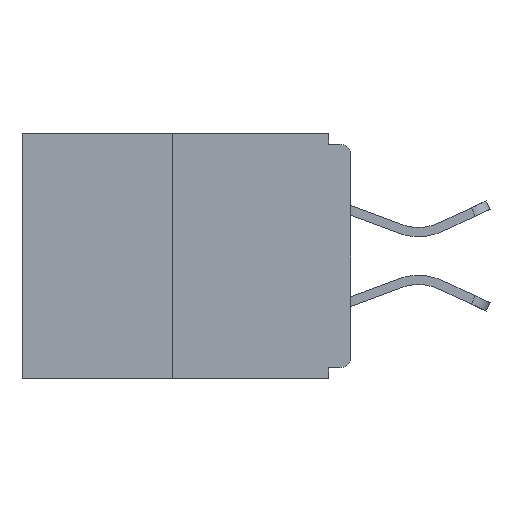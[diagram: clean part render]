
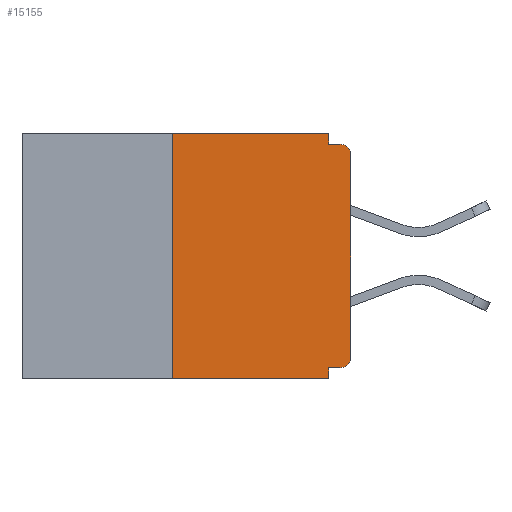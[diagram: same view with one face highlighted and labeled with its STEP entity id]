
A CAD part, left-side view. The second image highlights one B-rep face of the part: STEP entity #15155.
In plain terms, the highlighted planar face has unit normal (-1, 0, 0).
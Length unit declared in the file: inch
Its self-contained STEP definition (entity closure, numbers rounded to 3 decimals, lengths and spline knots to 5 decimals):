
#83 = CARTESIAN_POINT ( 'NONE',  ( 0., 0.015, -0.03 ) ) ;
#895 = CARTESIAN_POINT ( 'NONE',  ( 0., 0.46, 0. ) ) ;
#1027 = VECTOR ( 'NONE', #2472, 39.37008 ) ;
#1041 = VERTEX_POINT ( 'NONE', #11743 ) ;
#1158 = CARTESIAN_POINT ( 'NONE',  ( 0., 0.015, -0.328 ) ) ;
#1202 = FACE_OUTER_BOUND ( 'NONE', #19385, .T. ) ;
#1250 = LINE ( 'NONE', #4895, #5093 ) ;
#1972 = EDGE_CURVE ( 'NONE', #18766, #8095, #3754, .T. ) ;
#2022 = DIRECTION ( 'NONE',  ( -1., 0., 0. ) ) ;
#2089 = VECTOR ( 'NONE', #27656, 39.37008 ) ;
#2280 = ORIENTED_EDGE ( 'NONE', *, *, #21672, .F. ) ;
#2422 = DIRECTION ( 'NONE',  ( 0., 0., -1. ) ) ;
#2425 = LINE ( 'NONE', #4807, #1027 ) ;
#2444 = AXIS2_PLACEMENT_3D ( 'NONE', #895, #22980, #5081 ) ;
#2463 = VECTOR ( 'NONE', #12891, 39.37008 ) ;
#2472 = DIRECTION ( 'NONE',  ( 0., 0., 1. ) ) ;
#2702 = CARTESIAN_POINT ( 'NONE',  ( 0., 0., 0. ) ) ;
#3128 = PLANE ( 'NONE',  #2444 ) ;
#3177 = VECTOR ( 'NONE', #22020, 39.37008 ) ;
#3754 = LINE ( 'NONE', #13564, #22921 ) ;
#3843 = VECTOR ( 'NONE', #13869, 39.37008 ) ;
#3879 = ORIENTED_EDGE ( 'NONE', *, *, #1972, .F. ) ;
#4583 = ORIENTED_EDGE ( 'NONE', *, *, #4983, .F. ) ;
#4733 = CARTESIAN_POINT ( 'NONE',  ( 0., 0., -0.03 ) ) ;
#4807 = CARTESIAN_POINT ( 'NONE',  ( 0., 0.25, 0. ) ) ;
#4895 = CARTESIAN_POINT ( 'NONE',  ( 0., 0., -0.015 ) ) ;
#4983 = EDGE_CURVE ( 'NONE', #16900, #11001, #2425, .T. ) ;
#5081 = DIRECTION ( 'NONE',  ( 0., 0., -1. ) ) ;
#5093 = VECTOR ( 'NONE', #20841, 39.37008 ) ;
#5510 = DIRECTION ( 'NONE',  ( 0., 0., -1. ) ) ;
#5791 = VERTEX_POINT ( 'NONE', #23379 ) ;
#6194 = CARTESIAN_POINT ( 'NONE',  ( 0., 0.46, 0. ) ) ;
#7179 = CARTESIAN_POINT ( 'NONE',  ( 0., 0.031, -0.328 ) ) ;
#7752 = ORIENTED_EDGE ( 'NONE', *, *, #19307, .F. ) ;
#8095 = VERTEX_POINT ( 'NONE', #24979 ) ;
#8224 = ORIENTED_EDGE ( 'NONE', *, *, #23717, .T. ) ;
#8392 = CIRCLE ( 'NONE', #20581, 0.015 ) ;
#8876 = CARTESIAN_POINT ( 'NONE',  ( 0., 0.031, -0.343 ) ) ;
#9112 = LINE ( 'NONE', #8876, #3177 ) ;
#9368 = ORIENTED_EDGE ( 'NONE', *, *, #28503, .T. ) ;
#9593 = LINE ( 'NONE', #15163, #12023 ) ;
#9775 = LINE ( 'NONE', #2702, #3843 ) ;
#9916 = EDGE_CURVE ( 'NONE', #28762, #5791, #9112, .T. ) ;
#10580 = EDGE_CURVE ( 'NONE', #24247, #24507, #8392, .T. ) ;
#10732 = EDGE_CURVE ( 'NONE', #24507, #20897, #9775, .T. ) ;
#11001 = VERTEX_POINT ( 'NONE', #21272 ) ;
#11030 = ORIENTED_EDGE ( 'NONE', *, *, #10732, .T. ) ;
#11198 = EDGE_CURVE ( 'NONE', #11001, #18766, #16011, .T. ) ;
#11743 = CARTESIAN_POINT ( 'NONE',  ( 0., 0.015, -0.015 ) ) ;
#12023 = VECTOR ( 'NONE', #21525, 39.37008 ) ;
#12765 = ORIENTED_EDGE ( 'NONE', *, *, #11198, .F. ) ;
#12891 = DIRECTION ( 'NONE',  ( 0., -1., 0. ) ) ;
#13564 = CARTESIAN_POINT ( 'NONE',  ( 0., 0.031, 0. ) ) ;
#13869 = DIRECTION ( 'NONE',  ( 0., 0., 1. ) ) ;
#13969 = CARTESIAN_POINT ( 'NONE',  ( 0., 0., -0.313 ) ) ;
#15155 = ADVANCED_FACE ( 'NONE', ( #1202 ), #3128, .F. ) ;
#15163 = CARTESIAN_POINT ( 'NONE',  ( 0., 0.46, -0.343 ) ) ;
#16011 = LINE ( 'NONE', #6194, #2463 ) ;
#16308 = CIRCLE ( 'NONE', #18672, 0.015 ) ;
#16900 = VERTEX_POINT ( 'NONE', #24649 ) ;
#18611 = CARTESIAN_POINT ( 'NONE',  ( 0., 0., -0.328 ) ) ;
#18672 = AXIS2_PLACEMENT_3D ( 'NONE', #83, #24324, #22087 ) ;
#18766 = VERTEX_POINT ( 'NONE', #23336 ) ;
#19307 = EDGE_CURVE ( 'NONE', #24247, #28762, #25076, .T. ) ;
#19385 = EDGE_LOOP ( 'NONE', ( #12765, #4583, #8224, #24755, #7752, #22525, #11030, #9368, #2280, #3879 ) ) ;
#20217 = CARTESIAN_POINT ( 'NONE',  ( 0., 0.015, -0.313 ) ) ;
#20581 = AXIS2_PLACEMENT_3D ( 'NONE', #20217, #2022, #2422 ) ;
#20841 = DIRECTION ( 'NONE',  ( 0., -1., 0. ) ) ;
#20897 = VERTEX_POINT ( 'NONE', #4733 ) ;
#21272 = CARTESIAN_POINT ( 'NONE',  ( 0., 0.25, 0. ) ) ;
#21525 = DIRECTION ( 'NONE',  ( 0., -1., 0. ) ) ;
#21672 = EDGE_CURVE ( 'NONE', #8095, #1041, #1250, .T. ) ;
#22020 = DIRECTION ( 'NONE',  ( 0., 0., -1. ) ) ;
#22087 = DIRECTION ( 'NONE',  ( 0., 0., -1. ) ) ;
#22525 = ORIENTED_EDGE ( 'NONE', *, *, #10580, .T. ) ;
#22921 = VECTOR ( 'NONE', #5510, 39.37008 ) ;
#22980 = DIRECTION ( 'NONE',  ( 1., 0., 0. ) ) ;
#23336 = CARTESIAN_POINT ( 'NONE',  ( 0., 0.031, 0. ) ) ;
#23379 = CARTESIAN_POINT ( 'NONE',  ( 0., 0.031, -0.343 ) ) ;
#23717 = EDGE_CURVE ( 'NONE', #16900, #5791, #9593, .T. ) ;
#24247 = VERTEX_POINT ( 'NONE', #1158 ) ;
#24324 = DIRECTION ( 'NONE',  ( -1., 0., 0. ) ) ;
#24507 = VERTEX_POINT ( 'NONE', #13969 ) ;
#24649 = CARTESIAN_POINT ( 'NONE',  ( 0., 0.25, -0.343 ) ) ;
#24755 = ORIENTED_EDGE ( 'NONE', *, *, #9916, .F. ) ;
#24979 = CARTESIAN_POINT ( 'NONE',  ( 0., 0.031, -0.015 ) ) ;
#25076 = LINE ( 'NONE', #18611, #2089 ) ;
#27656 = DIRECTION ( 'NONE',  ( 0., 1., 0. ) ) ;
#28503 = EDGE_CURVE ( 'NONE', #20897, #1041, #16308, .T. ) ;
#28762 = VERTEX_POINT ( 'NONE', #7179 ) ;
